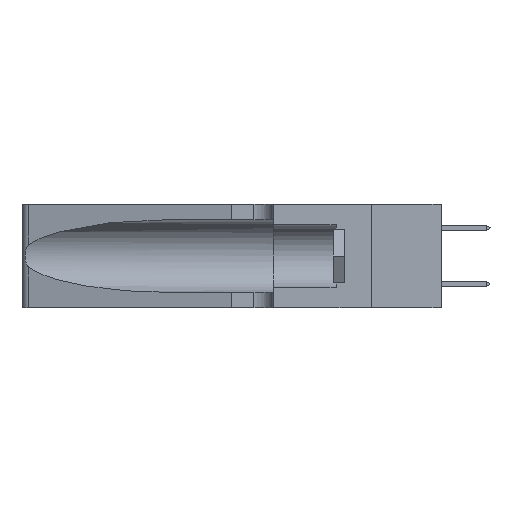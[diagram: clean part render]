
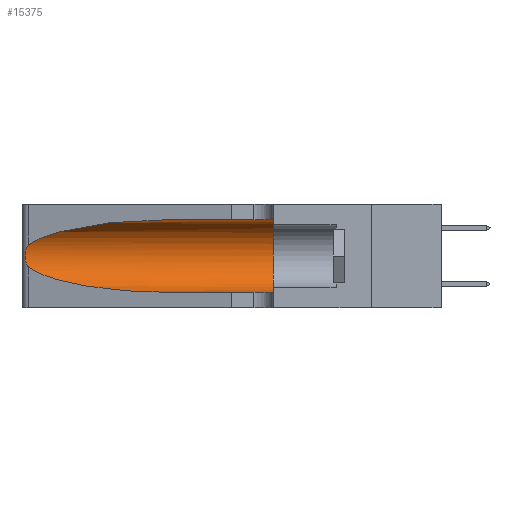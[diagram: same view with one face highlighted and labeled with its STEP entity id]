
A CAD part, left-side view. The second image highlights one B-rep face of the part: STEP entity #15375.
In plain terms, the highlighted cylindrical face has radius 3.308 mm (diameter 6.617 mm), a partial arc.
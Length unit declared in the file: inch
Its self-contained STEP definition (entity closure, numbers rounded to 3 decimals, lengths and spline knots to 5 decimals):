
#802 = VERTEX_POINT ( 'NONE', #26201 ) ;
#1366 = CARTESIAN_POINT ( 'NONE',  ( 0.18966, 0.96281, 0.05475 ) ) ;
#1625 = CARTESIAN_POINT ( 'NONE',  ( 0.25856, 1.23593, 0.16098 ) ) ;
#2337 = VERTEX_POINT ( 'NONE', #26704 ) ;
#4369 = CARTESIAN_POINT ( 'NONE',  ( 0.25555, 1.22993, 0.14849 ) ) ;
#4488 = CARTESIAN_POINT ( 'NONE',  ( 0.25639, 1.23186, 0.15144 ) ) ;
#4985 = CARTESIAN_POINT ( 'NONE',  ( 0.25487, 1.22718, 0.14631 ) ) ;
#5304 = CARTESIAN_POINT ( 'NONE',  ( 0.1305, 0.35, 0.185 ) ) ;
#6989 = CARTESIAN_POINT ( 'NONE',  ( 0.1305, 0.35, 0.05475 ) ) ;
#7106 = CARTESIAN_POINT ( 'NONE',  ( 0.25487, 1.22718, 0.14631 ) ) ;
#7220 = CARTESIAN_POINT ( 'NONE',  ( 0.26075, 1.23896, 0.19203 ) ) ;
#7251 = CARTESIAN_POINT ( 'NONE',  ( 0.18966, 0.96281, 0.31525 ) ) ;
#7283 = CARTESIAN_POINT ( 'NONE',  ( 0.1305, 0.35, 0.31525 ) ) ;
#7560 = CARTESIAN_POINT ( 'NONE',  ( 0.26018, 1.23835, 0.19895 ) ) ;
#7885 = B_SPLINE_CURVE_WITH_KNOTS ( 'NONE', 3,
 ( #34329, #17939, #15537, #20740, #12679, #7560, #7220, #23594, #26571, #1625, #20633, #4488, #4369, #7106 ),
 .UNSPECIFIED., .F., .F.,
 ( 4, 2, 2, 2, 2, 2, 4 ),
 ( 0., 0.00027, 0.00053, 0.00107, 0.0016, 0.00187, 0.00214 ),
 .UNSPECIFIED. ) ;
#8143 = CARTESIAN_POINT ( 'NONE',  ( 0.1305, 1.61858, 0.185 ) ) ;
#8247 = EDGE_CURVE ( 'NONE', #2337, #22942, #29415, .T. ) ;
#8745 = VERTEX_POINT ( 'NONE', #4985 ) ;
#10272 = VECTOR ( 'NONE', #22113, 39.37008 ) ;
#11263 = ORIENTED_EDGE ( 'NONE', *, *, #28433, .T. ) ;
#11814 = EDGE_CURVE ( 'NONE', #30803, #8745, #7885, .T. ) ;
#12679 = CARTESIAN_POINT ( 'NONE',  ( 0.25854, 1.2359, 0.20912 ) ) ;
#13057 = EDGE_CURVE ( 'NONE', #2337, #30803, #32068, .T. ) ;
#13706 = VERTEX_POINT ( 'NONE', #6989 ) ;
#13727 = CARTESIAN_POINT ( 'NONE',  ( 0.1305, 1.61858, 0.31525 ) ) ;
#14130 = ORIENTED_EDGE ( 'NONE', *, *, #17478, .T. ) ;
#14918 = EDGE_LOOP ( 'NONE', ( #16093, #32889, #11263, #14130, #32409, #34730 ) ) ;
#15375 = ADVANCED_FACE ( 'NONE', ( #26208 ), #28311, .F. ) ;
#15393 = CARTESIAN_POINT ( 'NONE',  ( 0.2373, 1.15595, 0.08982 ) ) ;
#15537 = CARTESIAN_POINT ( 'NONE',  ( 0.25639, 1.23184, 0.21858 ) ) ;
#15712 = VECTOR ( 'NONE', #28954, 39.37008 ) ;
#16093 = ORIENTED_EDGE ( 'NONE', *, *, #13057, .T. ) ;
#16386 =( BOUNDED_CURVE ( )  B_SPLINE_CURVE ( 3, ( #31430, #15393, #1366, #25974 ),
 .UNSPECIFIED., .F., .T. ) 
 B_SPLINE_CURVE_WITH_KNOTS ( ( 4, 4 ),
 ( 3.44316, 4.71239 ),
 .UNSPECIFIED. ) 
 CURVE ( )  GEOMETRIC_REPRESENTATION_ITEM ( )  RATIONAL_B_SPLINE_CURVE ( ( 1., 0.87, 0.87, 1. ) ) 
 REPRESENTATION_ITEM ( '' )  );
#17214 = EDGE_CURVE ( 'NONE', #22942, #13706, #22498, .T. ) ;
#17478 = EDGE_CURVE ( 'NONE', #802, #13706, #33596, .T. ) ;
#17745 = CARTESIAN_POINT ( 'NONE',  ( 0.1305, 0.72297, 0.31525 ) ) ;
#17939 = CARTESIAN_POINT ( 'NONE',  ( 0.25555, 1.22994, 0.2215 ) ) ;
#18293 = AXIS2_PLACEMENT_3D ( 'NONE', #5304, #32739, #21782 ) ;
#18318 = CARTESIAN_POINT ( 'NONE',  ( 0.25487, 1.22718, 0.22369 ) ) ;
#20436 = CARTESIAN_POINT ( 'NONE',  ( 0.2373, 1.15595, 0.28018 ) ) ;
#20633 = CARTESIAN_POINT ( 'NONE',  ( 0.25789, 1.23486, 0.15765 ) ) ;
#20659 = CARTESIAN_POINT ( 'NONE',  ( 0.25487, 1.22718, 0.22369 ) ) ;
#20740 = CARTESIAN_POINT ( 'NONE',  ( 0.25787, 1.23484, 0.2124 ) ) ;
#21782 = DIRECTION ( 'NONE',  ( 0., 0., 1. ) ) ;
#22113 = DIRECTION ( 'NONE',  ( 0., -1., 0. ) ) ;
#22498 = CIRCLE ( 'NONE', #18293, 0.13025 ) ;
#22942 = VERTEX_POINT ( 'NONE', #7283 ) ;
#23594 = CARTESIAN_POINT ( 'NONE',  ( 0.26075, 1.23896, 0.178 ) ) ;
#25974 = CARTESIAN_POINT ( 'NONE',  ( 0.1305, 0.72297, 0.05475 ) ) ;
#26201 = CARTESIAN_POINT ( 'NONE',  ( 0.1305, 0.72297, 0.05475 ) ) ;
#26208 = FACE_OUTER_BOUND ( 'NONE', #14918, .T. ) ;
#26571 = CARTESIAN_POINT ( 'NONE',  ( 0.26017, 1.23833, 0.17102 ) ) ;
#26704 = CARTESIAN_POINT ( 'NONE',  ( 0.1305, 0.72297, 0.31525 ) ) ;
#28311 = CYLINDRICAL_SURFACE ( 'NONE', #30493, 0.13025 ) ;
#28433 = EDGE_CURVE ( 'NONE', #8745, #802, #16386, .T. ) ;
#28954 = DIRECTION ( 'NONE',  ( 0., -1., 0. ) ) ;
#29415 = LINE ( 'NONE', #13727, #10272 ) ;
#29556 = DIRECTION ( 'NONE',  ( 0., -1., 0. ) ) ;
#30493 = AXIS2_PLACEMENT_3D ( 'NONE', #8143, #29556, #32509 ) ;
#30803 = VERTEX_POINT ( 'NONE', #18318 ) ;
#31430 = CARTESIAN_POINT ( 'NONE',  ( 0.25487, 1.22718, 0.14631 ) ) ;
#31435 = CARTESIAN_POINT ( 'NONE',  ( 0.1305, 1.61858, 0.05475 ) ) ;
#32068 =( BOUNDED_CURVE ( )  B_SPLINE_CURVE ( 3, ( #17745, #7251, #20436, #20659 ),
 .UNSPECIFIED., .F., .F. ) 
 B_SPLINE_CURVE_WITH_KNOTS ( ( 4, 4 ),
 ( 1.5708, 2.84003 ),
 .UNSPECIFIED. ) 
 CURVE ( )  GEOMETRIC_REPRESENTATION_ITEM ( )  RATIONAL_B_SPLINE_CURVE ( ( 1., 0.87, 0.87, 1. ) ) 
 REPRESENTATION_ITEM ( '' )  );
#32409 = ORIENTED_EDGE ( 'NONE', *, *, #17214, .F. ) ;
#32509 = DIRECTION ( 'NONE',  ( 0., 0., -1. ) ) ;
#32739 = DIRECTION ( 'NONE',  ( 0., 1., 0. ) ) ;
#32889 = ORIENTED_EDGE ( 'NONE', *, *, #11814, .T. ) ;
#33596 = LINE ( 'NONE', #31435, #15712 ) ;
#34329 = CARTESIAN_POINT ( 'NONE',  ( 0.25487, 1.22718, 0.22369 ) ) ;
#34730 = ORIENTED_EDGE ( 'NONE', *, *, #8247, .F. ) ;
